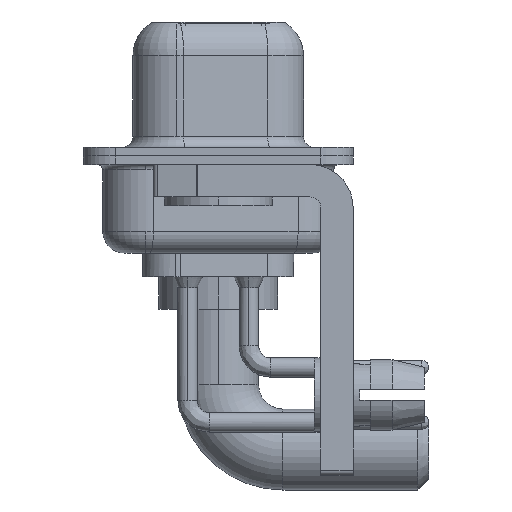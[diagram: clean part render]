
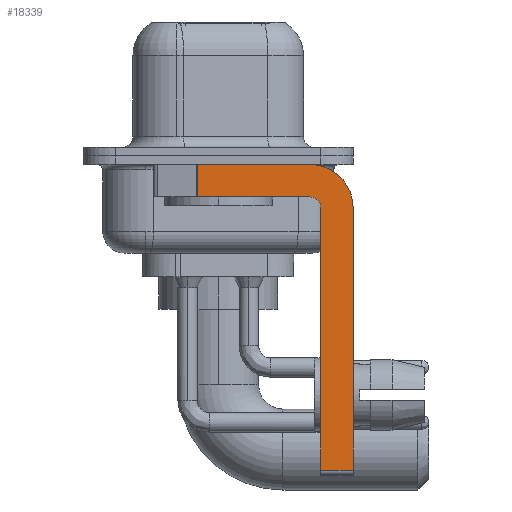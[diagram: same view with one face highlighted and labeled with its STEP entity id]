
A CAD part, left-side view. The second image highlights one B-rep face of the part: STEP entity #18339.
In plain terms, the highlighted planar face has unit normal (-1, 0, 0).
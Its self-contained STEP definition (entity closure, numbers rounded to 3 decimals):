
#12 = AXIS2_PLACEMENT_3D ( 'NONE', #14808, #3414, #3728 ) ;
#269 = CARTESIAN_POINT ( 'NONE',  ( -2.9, -4.25, -1.9 ) ) ;
#311 = CARTESIAN_POINT ( 'NONE',  ( -2.9, -4.75, -14.8 ) ) ;
#650 = EDGE_CURVE ( 'NONE', #16615, #5333, #14310, .T. ) ;
#892 = VECTOR ( 'NONE', #6418, 1000. ) ;
#1931 = LINE ( 'NONE', #16431, #892 ) ;
#2067 = VERTEX_POINT ( 'NONE', #8118 ) ;
#2134 = EDGE_CURVE ( 'NONE', #12421, #2166, #13135, .T. ) ;
#2166 = VERTEX_POINT ( 'NONE', #15047 ) ;
#2403 = EDGE_CURVE ( 'NONE', #13985, #13531, #9984, .T. ) ;
#2690 = LINE ( 'NONE', #14094, #12105 ) ;
#3414 = DIRECTION ( 'NONE',  ( 1., 0., 0. ) ) ;
#3728 = DIRECTION ( 'NONE',  ( 0., 0., -1. ) ) ;
#4004 = DIRECTION ( 'NONE',  ( 0., 0., 1. ) ) ;
#4020 = AXIS2_PLACEMENT_3D ( 'NONE', #18603, #20109, #4004 ) ;
#4789 = ORIENTED_EDGE ( 'NONE', *, *, #6436, .F. ) ;
#5017 = CARTESIAN_POINT ( 'NONE',  ( -2.9, -4.25, -14.55 ) ) ;
#5102 = DIRECTION ( 'NONE',  ( 0., 0., 1. ) ) ;
#5333 = VERTEX_POINT ( 'NONE', #15850 ) ;
#5724 = CARTESIAN_POINT ( 'NONE',  ( -2.9, -4.25, -2.4 ) ) ;
#6322 = VECTOR ( 'NONE', #16628, 1000. ) ;
#6418 = DIRECTION ( 'NONE',  ( 0., 0., -1. ) ) ;
#6436 = EDGE_CURVE ( 'NONE', #2067, #18189, #1931, .T. ) ;
#6709 = CIRCLE ( 'NONE', #7040, 2. ) ;
#6930 = LINE ( 'NONE', #5017, #6322 ) ;
#7029 = PLANE ( 'NONE',  #12 ) ;
#7040 = AXIS2_PLACEMENT_3D ( 'NONE', #5724, #18721, #14033 ) ;
#7217 = VECTOR ( 'NONE', #5102, 1000. ) ;
#7445 = EDGE_CURVE ( 'NONE', #16615, #2166, #2690, .T. ) ;
#7575 = VECTOR ( 'NONE', #10026, 1000. ) ;
#7810 = EDGE_CURVE ( 'NONE', #13985, #18189, #6930, .T. ) ;
#8091 = CARTESIAN_POINT ( 'NONE',  ( -2.9, -6.25, -14.55 ) ) ;
#8118 = CARTESIAN_POINT ( 'NONE',  ( -2.9, -6.25, -2.4 ) ) ;
#8427 = CIRCLE ( 'NONE', #4020, 0.5 ) ;
#9516 = ORIENTED_EDGE ( 'NONE', *, *, #14070, .F. ) ;
#9915 = CARTESIAN_POINT ( 'NONE',  ( -2.9, -4.25, -1.9 ) ) ;
#9984 = LINE ( 'NONE', #311, #7217 ) ;
#10026 = DIRECTION ( 'NONE',  ( 0., 1., 0. ) ) ;
#10099 = EDGE_CURVE ( 'NONE', #13531, #12421, #8427, .T. ) ;
#11281 = VECTOR ( 'NONE', #19111, 1000. ) ;
#12105 = VECTOR ( 'NONE', #17378, 1000. ) ;
#12421 = VERTEX_POINT ( 'NONE', #269 ) ;
#13062 = EDGE_LOOP ( 'NONE', ( #16468, #15723, #17824, #18374, #20526, #19027, #4789, #9516 ) ) ;
#13135 = LINE ( 'NONE', #9915, #7575 ) ;
#13311 = CARTESIAN_POINT ( 'NONE',  ( -2.9, -4.75, -2.4 ) ) ;
#13531 = VERTEX_POINT ( 'NONE', #13311 ) ;
#13985 = VERTEX_POINT ( 'NONE', #18292 ) ;
#14033 = DIRECTION ( 'NONE',  ( 0., 0., -1. ) ) ;
#14070 = EDGE_CURVE ( 'NONE', #5333, #2067, #6709, .T. ) ;
#14094 = CARTESIAN_POINT ( 'NONE',  ( -2.9, 0.978, -1.9 ) ) ;
#14310 = LINE ( 'NONE', #15811, #11281 ) ;
#14808 = CARTESIAN_POINT ( 'NONE',  ( -2.9, -4.25, -2.4 ) ) ;
#15019 = FACE_OUTER_BOUND ( 'NONE', #13062, .T. ) ;
#15047 = CARTESIAN_POINT ( 'NONE',  ( -2.9, 0.978, -1.9 ) ) ;
#15723 = ORIENTED_EDGE ( 'NONE', *, *, #7445, .T. ) ;
#15811 = CARTESIAN_POINT ( 'NONE',  ( -2.9, 3., -0.4 ) ) ;
#15850 = CARTESIAN_POINT ( 'NONE',  ( -2.9, -4.25, -0.4 ) ) ;
#16431 = CARTESIAN_POINT ( 'NONE',  ( -2.9, -6.25, -2.4 ) ) ;
#16468 = ORIENTED_EDGE ( 'NONE', *, *, #650, .F. ) ;
#16615 = VERTEX_POINT ( 'NONE', #18666 ) ;
#16628 = DIRECTION ( 'NONE',  ( 0., -1., 0. ) ) ;
#17378 = DIRECTION ( 'NONE',  ( 0., 0., -1. ) ) ;
#17824 = ORIENTED_EDGE ( 'NONE', *, *, #2134, .F. ) ;
#18189 = VERTEX_POINT ( 'NONE', #8091 ) ;
#18292 = CARTESIAN_POINT ( 'NONE',  ( -2.9, -4.75, -14.55 ) ) ;
#18339 = ADVANCED_FACE ( 'NONE', ( #15019 ), #7029, .F. ) ;
#18374 = ORIENTED_EDGE ( 'NONE', *, *, #10099, .F. ) ;
#18603 = CARTESIAN_POINT ( 'NONE',  ( -2.9, -4.25, -2.4 ) ) ;
#18666 = CARTESIAN_POINT ( 'NONE',  ( -2.9, 0.978, -0.4 ) ) ;
#18721 = DIRECTION ( 'NONE',  ( 1., 0., 0. ) ) ;
#19027 = ORIENTED_EDGE ( 'NONE', *, *, #7810, .T. ) ;
#19111 = DIRECTION ( 'NONE',  ( 0., -1., 0. ) ) ;
#20109 = DIRECTION ( 'NONE',  ( -1., 0., 0. ) ) ;
#20526 = ORIENTED_EDGE ( 'NONE', *, *, #2403, .F. ) ;
